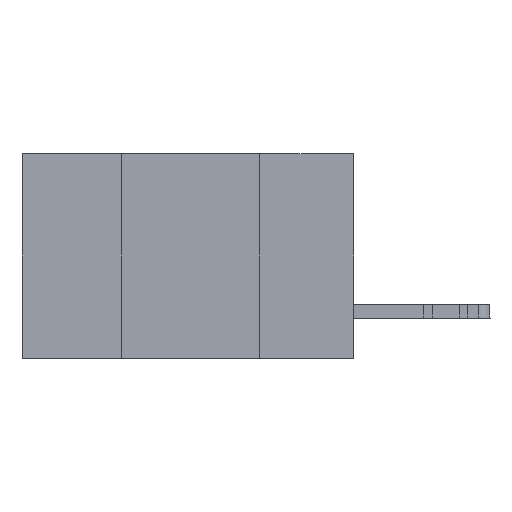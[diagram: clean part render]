
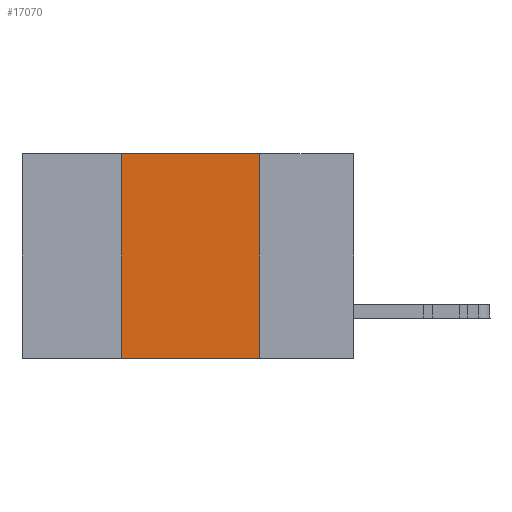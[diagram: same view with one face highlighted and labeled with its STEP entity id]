
A CAD part, left-side view. The second image highlights one B-rep face of the part: STEP entity #17070.
In plain terms, the highlighted planar face has unit normal (-1, 0, 0).
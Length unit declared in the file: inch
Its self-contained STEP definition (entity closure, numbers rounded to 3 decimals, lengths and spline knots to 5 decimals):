
#327 = CARTESIAN_POINT ( 'NONE',  ( 0., 0.42, -0.37 ) ) ;
#371 = LINE ( 'NONE', #42754, #15419 ) ;
#1475 = VERTEX_POINT ( 'NONE', #327 ) ;
#5791 = AXIS2_PLACEMENT_3D ( 'NONE', #45423, #37388, #10620 ) ;
#7663 = FACE_OUTER_BOUND ( 'NONE', #46654, .T. ) ;
#10466 = CARTESIAN_POINT ( 'NONE',  ( 0., 0.42, 0. ) ) ;
#10620 = DIRECTION ( 'NONE',  ( 0., 0., -1. ) ) ;
#11118 = DIRECTION ( 'NONE',  ( 0., 0., -1. ) ) ;
#13127 = ORIENTED_EDGE ( 'NONE', *, *, #45975, .F. ) ;
#13787 = EDGE_CURVE ( 'NONE', #35852, #18046, #48790, .T. ) ;
#14186 = CARTESIAN_POINT ( 'NONE',  ( 0., 0.17, 0. ) ) ;
#15419 = VECTOR ( 'NONE', #16713, 39.37008 ) ;
#16713 = DIRECTION ( 'NONE',  ( 0., 0., 1. ) ) ;
#17070 = ADVANCED_FACE ( 'NONE', ( #7663 ), #44721, .F. ) ;
#18046 = VERTEX_POINT ( 'NONE', #14186 ) ;
#19919 = ORIENTED_EDGE ( 'NONE', *, *, #46102, .T. ) ;
#20259 = CARTESIAN_POINT ( 'NONE',  ( 0., 0.6, -0.37 ) ) ;
#20554 = DIRECTION ( 'NONE',  ( 0., -1., 0. ) ) ;
#24136 = EDGE_CURVE ( 'NONE', #18046, #46258, #48989, .T. ) ;
#28164 = VECTOR ( 'NONE', #20554, 39.37008 ) ;
#28899 = ORIENTED_EDGE ( 'NONE', *, *, #13787, .F. ) ;
#33438 = VECTOR ( 'NONE', #11118, 39.37008 ) ;
#34045 = CARTESIAN_POINT ( 'NONE',  ( 0., 0.17, 0. ) ) ;
#34118 = VECTOR ( 'NONE', #36387, 39.37008 ) ;
#35852 = VERTEX_POINT ( 'NONE', #10466 ) ;
#36387 = DIRECTION ( 'NONE',  ( 0., -1., 0. ) ) ;
#37388 = DIRECTION ( 'NONE',  ( 1., 0., 0. ) ) ;
#37630 = CARTESIAN_POINT ( 'NONE',  ( 0., 0.17, -0.37 ) ) ;
#39935 = LINE ( 'NONE', #20259, #34118 ) ;
#42754 = CARTESIAN_POINT ( 'NONE',  ( 0., 0.42, 0. ) ) ;
#44721 = PLANE ( 'NONE',  #5791 ) ;
#45423 = CARTESIAN_POINT ( 'NONE',  ( 0., 0.6, 0. ) ) ;
#45975 = EDGE_CURVE ( 'NONE', #1475, #35852, #371, .T. ) ;
#46102 = EDGE_CURVE ( 'NONE', #1475, #46258, #39935, .T. ) ;
#46258 = VERTEX_POINT ( 'NONE', #37630 ) ;
#46654 = EDGE_LOOP ( 'NONE', ( #48525, #28899, #13127, #19919 ) ) ;
#46922 = CARTESIAN_POINT ( 'NONE',  ( 0., 0.6, 0. ) ) ;
#48525 = ORIENTED_EDGE ( 'NONE', *, *, #24136, .F. ) ;
#48790 = LINE ( 'NONE', #46922, #28164 ) ;
#48989 = LINE ( 'NONE', #34045, #33438 ) ;
